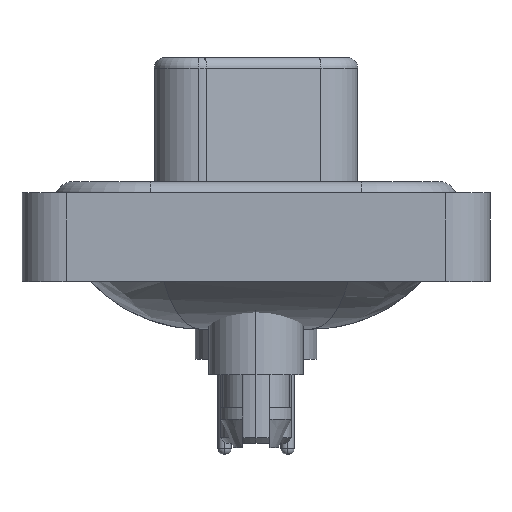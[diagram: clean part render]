
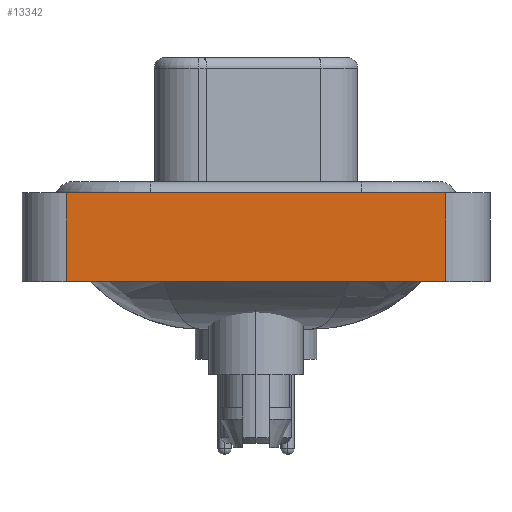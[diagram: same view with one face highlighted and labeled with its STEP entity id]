
A CAD part, left-side view. The second image highlights one B-rep face of the part: STEP entity #13342.
In plain terms, the highlighted planar face has unit normal (-1, 0, 0).
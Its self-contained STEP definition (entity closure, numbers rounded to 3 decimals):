
#354 = EDGE_CURVE ( 'NONE', #1660, #11529, #6424, .T. ) ;
#728 = DIRECTION ( 'NONE',  ( 0., -1., 0. ) ) ;
#751 = CARTESIAN_POINT ( 'NONE',  ( -7.35, -8.55, -3.6 ) ) ;
#1499 = DIRECTION ( 'NONE',  ( 0., 0., 1. ) ) ;
#1571 = DIRECTION ( 'NONE',  ( 0., -1., 0. ) ) ;
#1607 = DIRECTION ( 'NONE',  ( 0., 0., 1. ) ) ;
#1660 = VERTEX_POINT ( 'NONE', #8032 ) ;
#1813 = PLANE ( 'NONE',  #11309 ) ;
#2622 = ORIENTED_EDGE ( 'NONE', *, *, #14901, .T. ) ;
#3513 = VERTEX_POINT ( 'NONE', #15049 ) ;
#4743 = LINE ( 'NONE', #7815, #15640 ) ;
#4792 = CARTESIAN_POINT ( 'NONE',  ( -7.35, 8.55, -3.6 ) ) ;
#5869 = LINE ( 'NONE', #15737, #9506 ) ;
#6424 = LINE ( 'NONE', #4792, #6799 ) ;
#6473 = VERTEX_POINT ( 'NONE', #751 ) ;
#6527 = LINE ( 'NONE', #13218, #14892 ) ;
#6799 = VECTOR ( 'NONE', #1499, 1000. ) ;
#6858 = EDGE_CURVE ( 'NONE', #11529, #3513, #5869, .T. ) ;
#7815 = CARTESIAN_POINT ( 'NONE',  ( -7.35, -8.55, -3.6 ) ) ;
#8032 = CARTESIAN_POINT ( 'NONE',  ( -7.35, 8.55, -3.6 ) ) ;
#8293 = EDGE_LOOP ( 'NONE', ( #19886, #19510, #21517, #2622 ) ) ;
#9506 = VECTOR ( 'NONE', #728, 1000. ) ;
#10459 = FACE_OUTER_BOUND ( 'NONE', #8293, .T. ) ;
#11309 = AXIS2_PLACEMENT_3D ( 'NONE', #20108, #13650, #20310 ) ;
#11529 = VERTEX_POINT ( 'NONE', #21535 ) ;
#13218 = CARTESIAN_POINT ( 'NONE',  ( -7.35, -8.55, -3.6 ) ) ;
#13342 = ADVANCED_FACE ( 'NONE', ( #10459 ), #1813, .T. ) ;
#13650 = DIRECTION ( 'NONE',  ( -1., 0., 0. ) ) ;
#14412 = EDGE_CURVE ( 'NONE', #6473, #3513, #6527, .T. ) ;
#14892 = VECTOR ( 'NONE', #1607, 1000. ) ;
#14901 = EDGE_CURVE ( 'NONE', #1660, #6473, #4743, .T. ) ;
#15049 = CARTESIAN_POINT ( 'NONE',  ( -7.35, -8.55, 0.4 ) ) ;
#15640 = VECTOR ( 'NONE', #1571, 1000. ) ;
#15737 = CARTESIAN_POINT ( 'NONE',  ( -7.35, -8.55, 0.4 ) ) ;
#19510 = ORIENTED_EDGE ( 'NONE', *, *, #6858, .F. ) ;
#19886 = ORIENTED_EDGE ( 'NONE', *, *, #14412, .T. ) ;
#20108 = CARTESIAN_POINT ( 'NONE',  ( -7.35, -8.55, -3.6 ) ) ;
#20310 = DIRECTION ( 'NONE',  ( 0., 0., 1. ) ) ;
#21517 = ORIENTED_EDGE ( 'NONE', *, *, #354, .F. ) ;
#21535 = CARTESIAN_POINT ( 'NONE',  ( -7.35, 8.55, 0.4 ) ) ;
